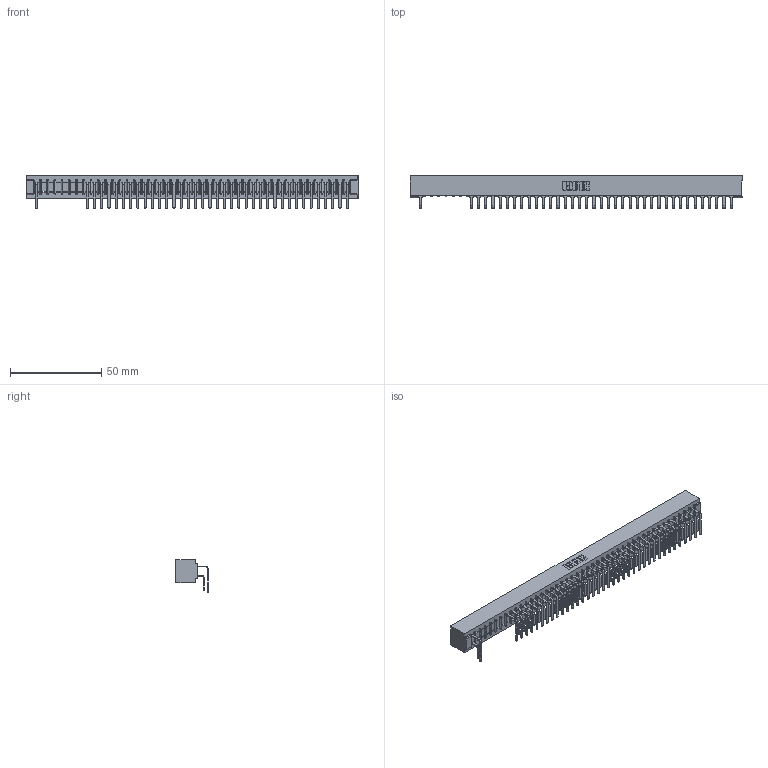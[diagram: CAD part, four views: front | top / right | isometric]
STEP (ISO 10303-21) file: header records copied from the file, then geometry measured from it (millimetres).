
FILE_DESCRIPTION (( 'STEP AP203' ), '1' );
FILE_NAME ('307-044-559-101.STEP', '2018-08-06T01:37:06', ( '' ), ( '' ), 'SwSTEP 2.0', 'SolidWorks 2016', '' );
FILE_SCHEMA (( 'CONFIG_CONTROL_DESIGN' ));
Length unit declared in the file: inch
Products named in the file (4): 307 Part_No Mounting Lugs; 307-290-001_558 559 - 1 (Single); 307-290-001_559 - 2 (Single); 307-044-559-101
Assembly tree (76 placements, depth 2):
  307-044-559-101
    307 Part_No Mounting Lugs
    307-290-001_558 559 - 1 (Single)  x37
    307-290-001_559 - 2 (Single)  x38
Bounding box: 182.22 x 17.69 x 18.07 mm (x, y, z)
Volume: 20104.5 mm3; surface area: 25796.8 mm2
Topology: 76 solids, 76 shells, 4035 faces, 11365 edges, 7354 vertices
Faces by surface type: plane 2619, cylinder 1326, sphere 90
Entity records: 39635 total; most frequent: CARTESIAN_POINT 6537, ORIENTED_EDGE 6490, DIRECTION 6387, EDGE_CURVE 3245, VECTOR 2491, LINE 2491, VERTEX_POINT 2098, AXIS2_PLACEMENT_3D 1948
